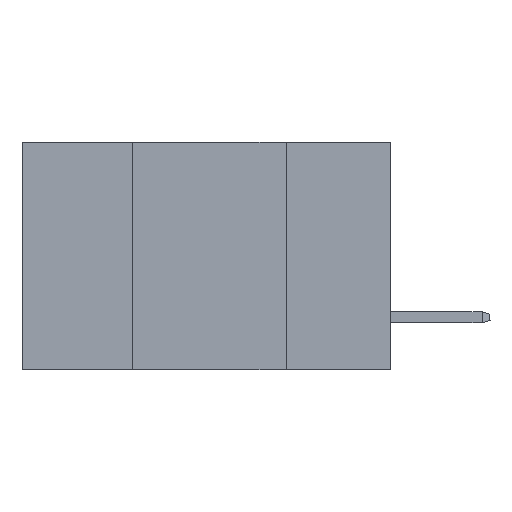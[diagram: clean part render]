
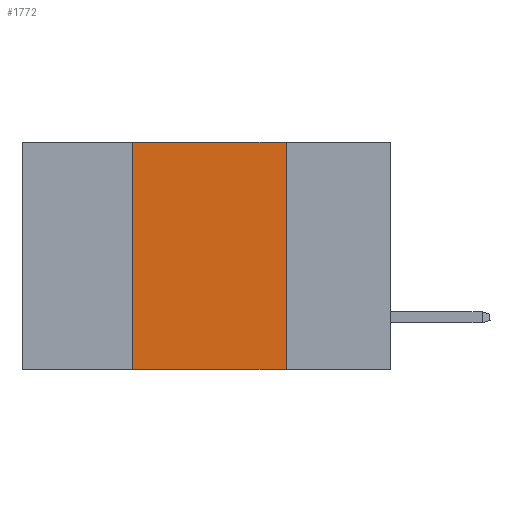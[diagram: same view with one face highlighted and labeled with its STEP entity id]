
A CAD part, left-side view. The second image highlights one B-rep face of the part: STEP entity #1772.
In plain terms, the highlighted planar face has unit normal (-1, 0, 0).
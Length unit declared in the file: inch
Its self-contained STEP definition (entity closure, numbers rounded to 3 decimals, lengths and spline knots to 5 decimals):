
#9 = DIRECTION ( 'NONE',  ( 1., 0., 0. ) ) ;
#47 = CARTESIAN_POINT ( 'NONE',  ( 0., 0.42, 0. ) ) ;
#1204 = DIRECTION ( 'NONE',  ( 0., 0., -1. ) ) ;
#1474 = EDGE_LOOP ( 'NONE', ( #7316, #9900, #13680, #17316 ) ) ;
#1630 = EDGE_CURVE ( 'NONE', #4991, #6626, #13292, .T. ) ;
#1772 = ADVANCED_FACE ( 'NONE', ( #16314 ), #27473, .F. ) ;
#2278 = VERTEX_POINT ( 'NONE', #25154 ) ;
#3055 = AXIS2_PLACEMENT_3D ( 'NONE', #25264, #9, #27396 ) ;
#3696 = EDGE_CURVE ( 'NONE', #6626, #4857, #5192, .T. ) ;
#4173 = CARTESIAN_POINT ( 'NONE',  ( 0., 0.6, 0. ) ) ;
#4514 = DIRECTION ( 'NONE',  ( 0., -1., 0. ) ) ;
#4857 = VERTEX_POINT ( 'NONE', #18147 ) ;
#4991 = VERTEX_POINT ( 'NONE', #18851 ) ;
#5192 = LINE ( 'NONE', #4173, #24499 ) ;
#5460 = EDGE_CURVE ( 'NONE', #4991, #2278, #6857, .T. ) ;
#5619 = VECTOR ( 'NONE', #12086, 39.37008 ) ;
#6087 = VECTOR ( 'NONE', #1204, 39.37008 ) ;
#6121 = DIRECTION ( 'NONE',  ( 0., -1., 0. ) ) ;
#6626 = VERTEX_POINT ( 'NONE', #47 ) ;
#6857 = LINE ( 'NONE', #8967, #16570 ) ;
#7316 = ORIENTED_EDGE ( 'NONE', *, *, #7782, .F. ) ;
#7782 = EDGE_CURVE ( 'NONE', #4857, #2278, #27368, .T. ) ;
#8967 = CARTESIAN_POINT ( 'NONE',  ( 0., 0.6, -0.37 ) ) ;
#9900 = ORIENTED_EDGE ( 'NONE', *, *, #3696, .F. ) ;
#12086 = DIRECTION ( 'NONE',  ( 0., 0., 1. ) ) ;
#13292 = LINE ( 'NONE', #24916, #5619 ) ;
#13680 = ORIENTED_EDGE ( 'NONE', *, *, #1630, .F. ) ;
#16314 = FACE_OUTER_BOUND ( 'NONE', #1474, .T. ) ;
#16570 = VECTOR ( 'NONE', #4514, 39.37008 ) ;
#17316 = ORIENTED_EDGE ( 'NONE', *, *, #5460, .T. ) ;
#18147 = CARTESIAN_POINT ( 'NONE',  ( 0., 0.17, 0. ) ) ;
#18851 = CARTESIAN_POINT ( 'NONE',  ( 0., 0.42, -0.37 ) ) ;
#24499 = VECTOR ( 'NONE', #6121, 39.37008 ) ;
#24554 = CARTESIAN_POINT ( 'NONE',  ( 0., 0.17, 0. ) ) ;
#24916 = CARTESIAN_POINT ( 'NONE',  ( 0., 0.42, 0. ) ) ;
#25154 = CARTESIAN_POINT ( 'NONE',  ( 0., 0.17, -0.37 ) ) ;
#25264 = CARTESIAN_POINT ( 'NONE',  ( 0., 0.6, 0. ) ) ;
#27368 = LINE ( 'NONE', #24554, #6087 ) ;
#27396 = DIRECTION ( 'NONE',  ( 0., 0., -1. ) ) ;
#27473 = PLANE ( 'NONE',  #3055 ) ;
